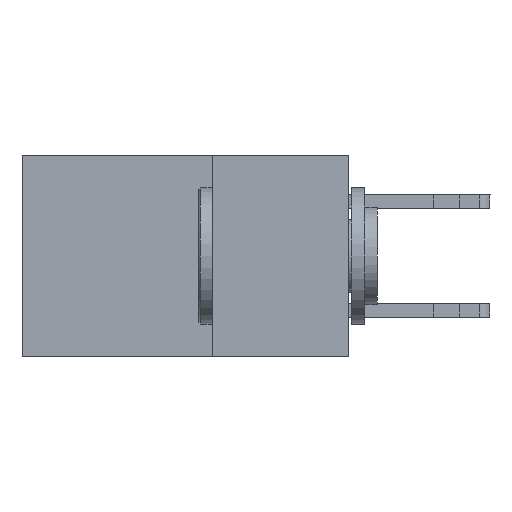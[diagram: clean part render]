
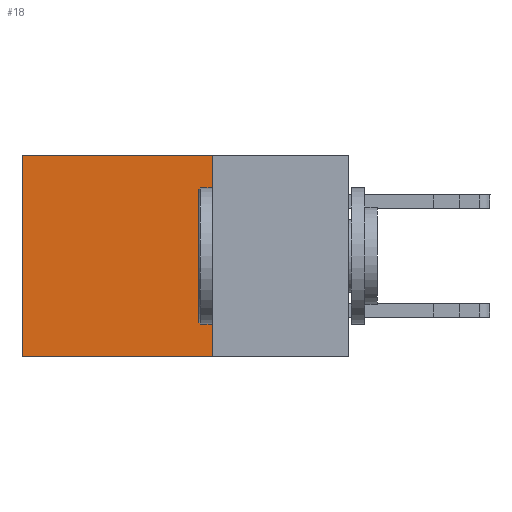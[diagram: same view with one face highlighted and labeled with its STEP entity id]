
A CAD part, left-side view. The second image highlights one B-rep face of the part: STEP entity #18.
In plain terms, the highlighted planar face has unit normal (-1, 0, 0).
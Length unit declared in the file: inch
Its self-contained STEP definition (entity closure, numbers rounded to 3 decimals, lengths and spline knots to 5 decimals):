
#18 = ADVANCED_FACE ( 'NONE', ( #11305 ), #272, .F. ) ;
#272 = PLANE ( 'NONE',  #15667 ) ;
#446 = CARTESIAN_POINT ( 'NONE',  ( 0.298, 0.25, 0. ) ) ;
#1543 = CARTESIAN_POINT ( 'NONE',  ( 0.298, 0.6, -0.37 ) ) ;
#1563 = VERTEX_POINT ( 'NONE', #3295 ) ;
#2844 = ORIENTED_EDGE ( 'NONE', *, *, #9668, .F. ) ;
#2874 = VERTEX_POINT ( 'NONE', #1543 ) ;
#3295 = CARTESIAN_POINT ( 'NONE',  ( 0.298, 0.25, 0. ) ) ;
#3657 = EDGE_CURVE ( 'NONE', #1563, #11894, #14970, .T. ) ;
#3964 = DIRECTION ( 'NONE',  ( 0., 0., -1. ) ) ;
#5068 = VECTOR ( 'NONE', #22589, 39.37008 ) ;
#5967 = CARTESIAN_POINT ( 'NONE',  ( 0.298, 0.25, 0. ) ) ;
#6058 = CARTESIAN_POINT ( 'NONE',  ( 0.298, 0.25, 0. ) ) ;
#6805 = CARTESIAN_POINT ( 'NONE',  ( 0.298, 0.25, -0.37 ) ) ;
#7330 = EDGE_CURVE ( 'NONE', #10550, #2874, #9843, .T. ) ;
#7707 = DIRECTION ( 'NONE',  ( 0., 1., 0. ) ) ;
#9496 = CARTESIAN_POINT ( 'NONE',  ( 0.298, 0.25, -0.37 ) ) ;
#9668 = EDGE_CURVE ( 'NONE', #11894, #2874, #18515, .T. ) ;
#9806 = CARTESIAN_POINT ( 'NONE',  ( 0.298, 0.6, 0. ) ) ;
#9843 = LINE ( 'NONE', #13657, #5068 ) ;
#10550 = VERTEX_POINT ( 'NONE', #9806 ) ;
#11094 = ORIENTED_EDGE ( 'NONE', *, *, #15312, .T. ) ;
#11305 = FACE_OUTER_BOUND ( 'NONE', #11684, .T. ) ;
#11684 = EDGE_LOOP ( 'NONE', ( #20171, #2844, #14981, #11094 ) ) ;
#11894 = VERTEX_POINT ( 'NONE', #6805 ) ;
#13331 = DIRECTION ( 'NONE',  ( 0., 0., -1. ) ) ;
#13563 = VECTOR ( 'NONE', #13331, 39.37008 ) ;
#13657 = CARTESIAN_POINT ( 'NONE',  ( 0.298, 0.6, 0. ) ) ;
#14675 = VECTOR ( 'NONE', #7707, 39.37008 ) ;
#14970 = LINE ( 'NONE', #6058, #13563 ) ;
#14981 = ORIENTED_EDGE ( 'NONE', *, *, #3657, .F. ) ;
#15312 = EDGE_CURVE ( 'NONE', #1563, #10550, #18502, .T. ) ;
#15667 = AXIS2_PLACEMENT_3D ( 'NONE', #5967, #18332, #3964 ) ;
#16614 = DIRECTION ( 'NONE',  ( 0., 1., 0. ) ) ;
#16735 = VECTOR ( 'NONE', #16614, 39.37008 ) ;
#18332 = DIRECTION ( 'NONE',  ( 1., 0., 0. ) ) ;
#18502 = LINE ( 'NONE', #446, #14675 ) ;
#18515 = LINE ( 'NONE', #9496, #16735 ) ;
#20171 = ORIENTED_EDGE ( 'NONE', *, *, #7330, .T. ) ;
#22589 = DIRECTION ( 'NONE',  ( 0., 0., -1. ) ) ;
